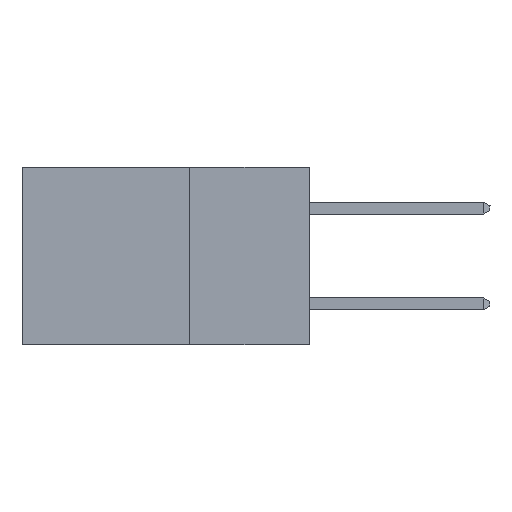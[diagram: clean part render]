
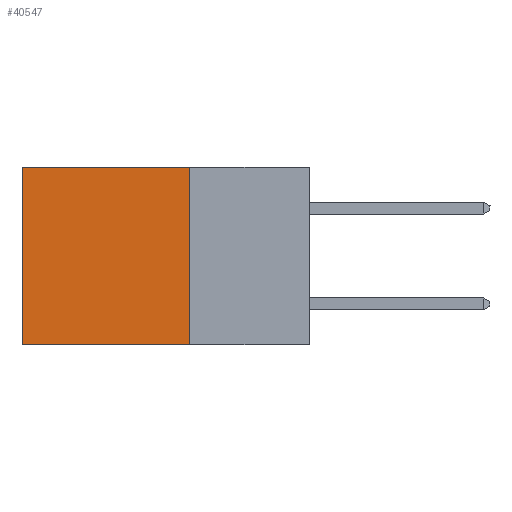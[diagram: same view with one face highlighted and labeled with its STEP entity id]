
A CAD part, left-side view. The second image highlights one B-rep face of the part: STEP entity #40547.
In plain terms, the highlighted planar face has unit normal (-1, 0, 0).
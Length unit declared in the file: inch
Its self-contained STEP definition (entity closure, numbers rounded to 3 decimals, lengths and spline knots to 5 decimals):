
#288 = FACE_OUTER_BOUND ( 'NONE', #6173, .T. ) ;
#316 = CARTESIAN_POINT ( 'NONE',  ( 0.2875, 0.25, -0.37 ) ) ;
#553 = DIRECTION ( 'NONE',  ( 0., 0., -1. ) ) ;
#626 = DIRECTION ( 'NONE',  ( 0., 1., 0. ) ) ;
#3647 = VECTOR ( 'NONE', #626, 39.37008 ) ;
#6173 = EDGE_LOOP ( 'NONE', ( #41537, #23046, #11191, #13955 ) ) ;
#7295 = CARTESIAN_POINT ( 'NONE',  ( 0.2875, 0.25, -0.37 ) ) ;
#7557 = CARTESIAN_POINT ( 'NONE',  ( 0.2875, 0.25, 0. ) ) ;
#7838 = CARTESIAN_POINT ( 'NONE',  ( 0.2875, 0.6, 0. ) ) ;
#8289 = EDGE_CURVE ( 'NONE', #13563, #41913, #8490, .T. ) ;
#8490 = LINE ( 'NONE', #30319, #35740 ) ;
#8686 = AXIS2_PLACEMENT_3D ( 'NONE', #7557, #21950, #553 ) ;
#10597 = CARTESIAN_POINT ( 'NONE',  ( 0.2875, 0.6, -0.37 ) ) ;
#11191 = ORIENTED_EDGE ( 'NONE', *, *, #17924, .F. ) ;
#13135 = LINE ( 'NONE', #316, #3647 ) ;
#13563 = VERTEX_POINT ( 'NONE', #38240 ) ;
#13955 = ORIENTED_EDGE ( 'NONE', *, *, #8289, .T. ) ;
#14336 = EDGE_CURVE ( 'NONE', #14836, #24187, #13135, .T. ) ;
#14836 = VERTEX_POINT ( 'NONE', #7295 ) ;
#15072 = VECTOR ( 'NONE', #32369, 39.37008 ) ;
#17924 = EDGE_CURVE ( 'NONE', #13563, #14836, #31701, .T. ) ;
#19649 = DIRECTION ( 'NONE',  ( 0., 1., 0. ) ) ;
#21950 = DIRECTION ( 'NONE',  ( 1., 0., 0. ) ) ;
#23046 = ORIENTED_EDGE ( 'NONE', *, *, #14336, .F. ) ;
#24187 = VERTEX_POINT ( 'NONE', #10597 ) ;
#28635 = EDGE_CURVE ( 'NONE', #41913, #24187, #38017, .T. ) ;
#28832 = CARTESIAN_POINT ( 'NONE',  ( 0.2875, 0.25, 0. ) ) ;
#29202 = DIRECTION ( 'NONE',  ( 0., 0., -1. ) ) ;
#30319 = CARTESIAN_POINT ( 'NONE',  ( 0.2875, 0.25, 0. ) ) ;
#31701 = LINE ( 'NONE', #28832, #15072 ) ;
#32369 = DIRECTION ( 'NONE',  ( 0., 0., -1. ) ) ;
#32457 = PLANE ( 'NONE',  #8686 ) ;
#35740 = VECTOR ( 'NONE', #19649, 39.37008 ) ;
#36930 = VECTOR ( 'NONE', #29202, 39.37008 ) ;
#38017 = LINE ( 'NONE', #7838, #36930 ) ;
#38240 = CARTESIAN_POINT ( 'NONE',  ( 0.2875, 0.25, 0. ) ) ;
#40547 = ADVANCED_FACE ( 'NONE', ( #288 ), #32457, .F. ) ;
#41537 = ORIENTED_EDGE ( 'NONE', *, *, #28635, .T. ) ;
#41913 = VERTEX_POINT ( 'NONE', #45847 ) ;
#45847 = CARTESIAN_POINT ( 'NONE',  ( 0.2875, 0.6, 0. ) ) ;
